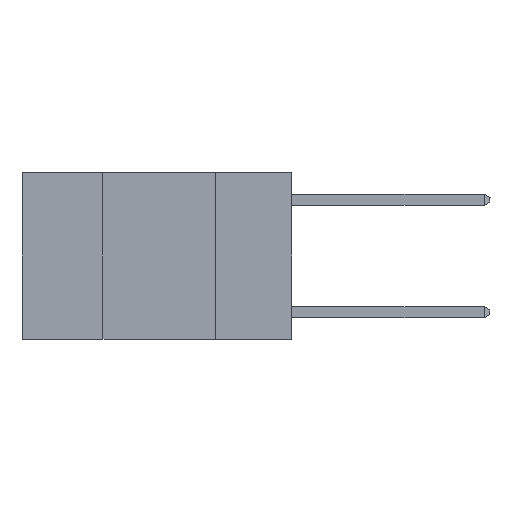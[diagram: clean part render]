
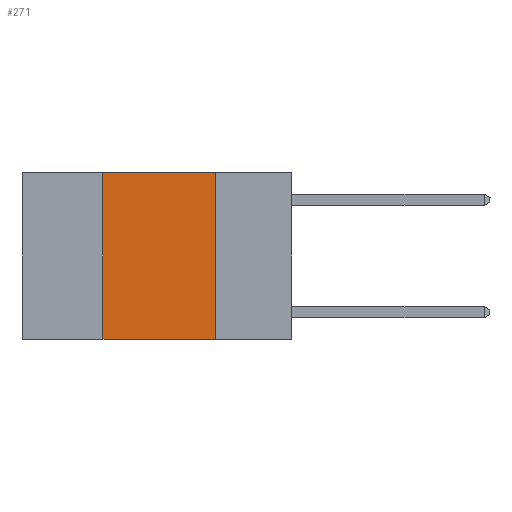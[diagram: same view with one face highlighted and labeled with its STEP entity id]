
A CAD part, left-side view. The second image highlights one B-rep face of the part: STEP entity #271.
In plain terms, the highlighted planar face has unit normal (-1, 0, 0).
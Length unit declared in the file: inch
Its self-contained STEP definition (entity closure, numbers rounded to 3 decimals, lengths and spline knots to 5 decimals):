
#36 = VERTEX_POINT ( 'NONE', #2198 ) ;
#271 = ADVANCED_FACE ( 'NONE', ( #1173 ), #4137, .F. ) ;
#1162 = VECTOR ( 'NONE', #4723, 39.37008 ) ;
#1173 = FACE_OUTER_BOUND ( 'NONE', #9384, .T. ) ;
#1523 = EDGE_CURVE ( 'NONE', #6962, #3415, #4140, .T. ) ;
#1539 = CARTESIAN_POINT ( 'NONE',  ( 0., 0.17, 0. ) ) ;
#2198 = CARTESIAN_POINT ( 'NONE',  ( 0., 0.17, -0.37 ) ) ;
#2361 = CARTESIAN_POINT ( 'NONE',  ( 0., 0.42, 0. ) ) ;
#2438 = ORIENTED_EDGE ( 'NONE', *, *, #6721, .T. ) ;
#2491 = VECTOR ( 'NONE', #8675, 39.37008 ) ;
#2741 = EDGE_CURVE ( 'NONE', #3415, #4611, #9419, .T. ) ;
#2745 = CARTESIAN_POINT ( 'NONE',  ( 0., 0.6, 0. ) ) ;
#2849 = CARTESIAN_POINT ( 'NONE',  ( 0., 0.42, -0.37 ) ) ;
#3195 = LINE ( 'NONE', #8365, #1162 ) ;
#3415 = VERTEX_POINT ( 'NONE', #9013 ) ;
#4137 = PLANE ( 'NONE',  #9579 ) ;
#4140 = LINE ( 'NONE', #2361, #6869 ) ;
#4313 = ORIENTED_EDGE ( 'NONE', *, *, #6146, .F. ) ;
#4389 = ORIENTED_EDGE ( 'NONE', *, *, #1523, .F. ) ;
#4611 = VERTEX_POINT ( 'NONE', #1539 ) ;
#4723 = DIRECTION ( 'NONE',  ( 0., -1., 0. ) ) ;
#5461 = DIRECTION ( 'NONE',  ( 1., 0., 0. ) ) ;
#5641 = DIRECTION ( 'NONE',  ( 0., 0., 1. ) ) ;
#6146 = EDGE_CURVE ( 'NONE', #4611, #36, #9100, .T. ) ;
#6721 = EDGE_CURVE ( 'NONE', #6962, #36, #3195, .T. ) ;
#6869 = VECTOR ( 'NONE', #5641, 39.37008 ) ;
#6962 = VERTEX_POINT ( 'NONE', #2849 ) ;
#8023 = VECTOR ( 'NONE', #8274, 39.37008 ) ;
#8274 = DIRECTION ( 'NONE',  ( 0., 0., -1. ) ) ;
#8365 = CARTESIAN_POINT ( 'NONE',  ( 0., 0.6, -0.37 ) ) ;
#8415 = DIRECTION ( 'NONE',  ( 0., 0., -1. ) ) ;
#8675 = DIRECTION ( 'NONE',  ( 0., -1., 0. ) ) ;
#9013 = CARTESIAN_POINT ( 'NONE',  ( 0., 0.42, 0. ) ) ;
#9058 = CARTESIAN_POINT ( 'NONE',  ( 0., 0.17, 0. ) ) ;
#9098 = CARTESIAN_POINT ( 'NONE',  ( 0., 0.6, 0. ) ) ;
#9100 = LINE ( 'NONE', #9058, #8023 ) ;
#9384 = EDGE_LOOP ( 'NONE', ( #4313, #9586, #4389, #2438 ) ) ;
#9419 = LINE ( 'NONE', #2745, #2491 ) ;
#9579 = AXIS2_PLACEMENT_3D ( 'NONE', #9098, #5461, #8415 ) ;
#9586 = ORIENTED_EDGE ( 'NONE', *, *, #2741, .F. ) ;
